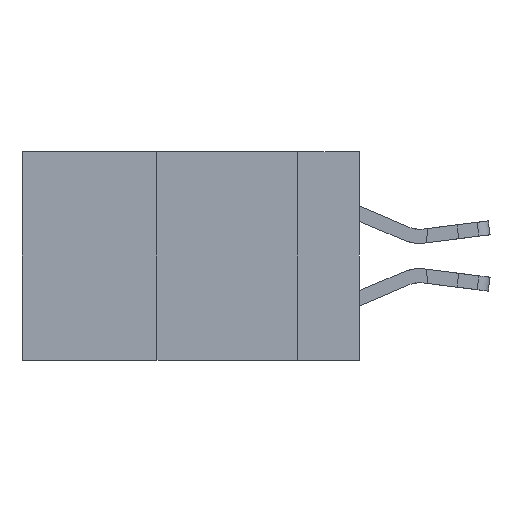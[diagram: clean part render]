
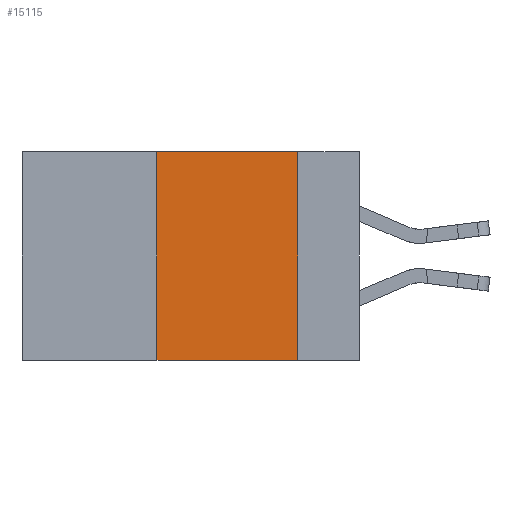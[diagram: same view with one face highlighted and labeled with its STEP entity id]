
A CAD part, left-side view. The second image highlights one B-rep face of the part: STEP entity #15115.
In plain terms, the highlighted planar face has unit normal (-1, 0, 0).
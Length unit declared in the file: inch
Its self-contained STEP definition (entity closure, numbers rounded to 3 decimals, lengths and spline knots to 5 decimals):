
#59 = DIRECTION ( 'NONE',  ( 1., 0., 0. ) ) ;
#179 = CARTESIAN_POINT ( 'NONE',  ( 0., 0.36, 0. ) ) ;
#240 = EDGE_CURVE ( 'NONE', #1453, #1778, #12995, .T. ) ;
#777 = CARTESIAN_POINT ( 'NONE',  ( 0., 0.11, 0. ) ) ;
#1430 = DIRECTION ( 'NONE',  ( 0., 0., -1. ) ) ;
#1453 = VERTEX_POINT ( 'NONE', #179 ) ;
#1778 = VERTEX_POINT ( 'NONE', #777 ) ;
#1976 = LINE ( 'NONE', #14597, #8672 ) ;
#2785 = LINE ( 'NONE', #10532, #13898 ) ;
#3121 = EDGE_CURVE ( 'NONE', #1778, #11298, #2785, .T. ) ;
#3276 = ORIENTED_EDGE ( 'NONE', *, *, #11703, .F. ) ;
#3641 = DIRECTION ( 'NONE',  ( 0., 0., -1. ) ) ;
#4150 = FACE_OUTER_BOUND ( 'NONE', #17556, .T. ) ;
#4653 = DIRECTION ( 'NONE',  ( 0., -1., 0. ) ) ;
#5746 = PLANE ( 'NONE',  #11318 ) ;
#5750 = VERTEX_POINT ( 'NONE', #16966 ) ;
#6460 = LINE ( 'NONE', #16035, #15674 ) ;
#6894 = CARTESIAN_POINT ( 'NONE',  ( 0., 0.6, 0. ) ) ;
#6984 = VECTOR ( 'NONE', #4653, 39.37008 ) ;
#7198 = CARTESIAN_POINT ( 'NONE',  ( 0., 0.11, -0.37 ) ) ;
#7691 = EDGE_CURVE ( 'NONE', #5750, #11298, #1976, .T. ) ;
#8098 = ORIENTED_EDGE ( 'NONE', *, *, #7691, .T. ) ;
#8672 = VECTOR ( 'NONE', #12437, 39.37008 ) ;
#10532 = CARTESIAN_POINT ( 'NONE',  ( 0., 0.11, 0. ) ) ;
#10601 = DIRECTION ( 'NONE',  ( 0., 0., 1. ) ) ;
#11298 = VERTEX_POINT ( 'NONE', #7198 ) ;
#11318 = AXIS2_PLACEMENT_3D ( 'NONE', #6894, #59, #1430 ) ;
#11703 = EDGE_CURVE ( 'NONE', #5750, #1453, #6460, .T. ) ;
#11910 = ORIENTED_EDGE ( 'NONE', *, *, #3121, .F. ) ;
#12437 = DIRECTION ( 'NONE',  ( 0., -1., 0. ) ) ;
#12995 = LINE ( 'NONE', #15726, #6984 ) ;
#13441 = ORIENTED_EDGE ( 'NONE', *, *, #240, .F. ) ;
#13898 = VECTOR ( 'NONE', #3641, 39.37008 ) ;
#14597 = CARTESIAN_POINT ( 'NONE',  ( 0., 0.6, -0.37 ) ) ;
#15115 = ADVANCED_FACE ( 'NONE', ( #4150 ), #5746, .F. ) ;
#15674 = VECTOR ( 'NONE', #10601, 39.37008 ) ;
#15726 = CARTESIAN_POINT ( 'NONE',  ( 0., 0.6, 0. ) ) ;
#16035 = CARTESIAN_POINT ( 'NONE',  ( 0., 0.36, 0. ) ) ;
#16966 = CARTESIAN_POINT ( 'NONE',  ( 0., 0.36, -0.37 ) ) ;
#17556 = EDGE_LOOP ( 'NONE', ( #11910, #13441, #3276, #8098 ) ) ;
